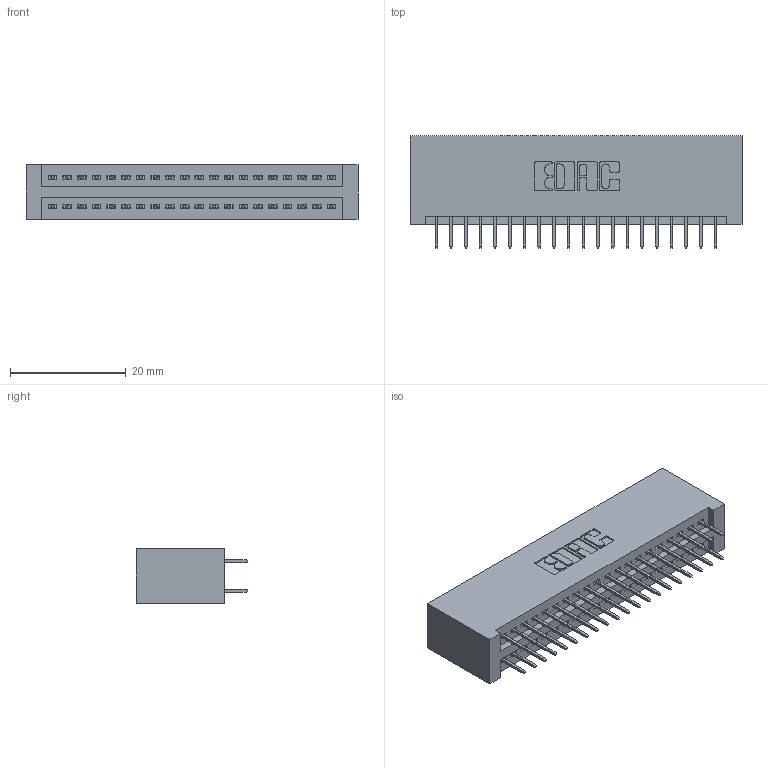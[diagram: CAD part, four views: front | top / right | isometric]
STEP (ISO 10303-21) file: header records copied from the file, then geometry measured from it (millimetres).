
FILE_DESCRIPTION (( 'STEP AP203' ), '1' );
FILE_NAME ('395-040-524-201.STEP', '2018-11-14T17:16:09', ( '' ), ( '' ), 'SwSTEP 2.0', 'SolidWorks 2016', '' );
FILE_SCHEMA (( 'CONFIG_CONTROL_DESIGN' ));
Length unit declared in the file: inch
Products named in the file (3): 345-292-001_345-293-124; 345 Part_No Mounting Lugs; 395-040-524-201
Assembly tree (41 placements, depth 2):
  395-040-524-201
    345 Part_No Mounting Lugs
    345-292-001_345-293-124  x40
Bounding box: 57.4 x 19.35 x 9.4 mm (x, y, z)
Volume: 5927.4 mm3; surface area: 8479.1 mm2
Topology: 41 solids, 41 shells, 2278 faces, 6437 edges, 4130 vertices
Faces by surface type: plane 1636, cylinder 642
Entity records: 18451 total; most frequent: CARTESIAN_POINT 3112, ORIENTED_EDGE 3046, DIRECTION 2767, EDGE_CURVE 1523, VECTOR 1323, LINE 1323, VERTEX_POINT 1010, AXIS2_PLACEMENT_3D 722
